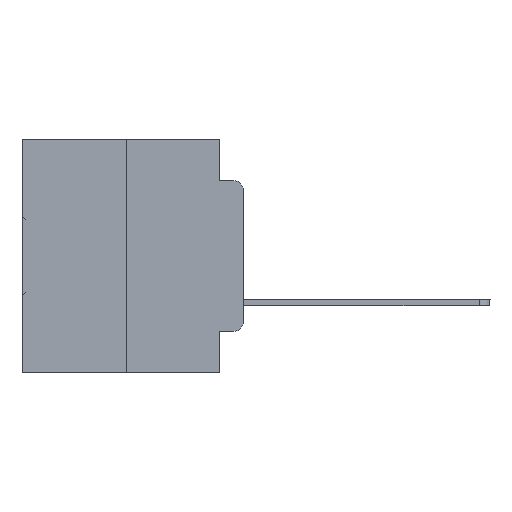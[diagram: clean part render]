
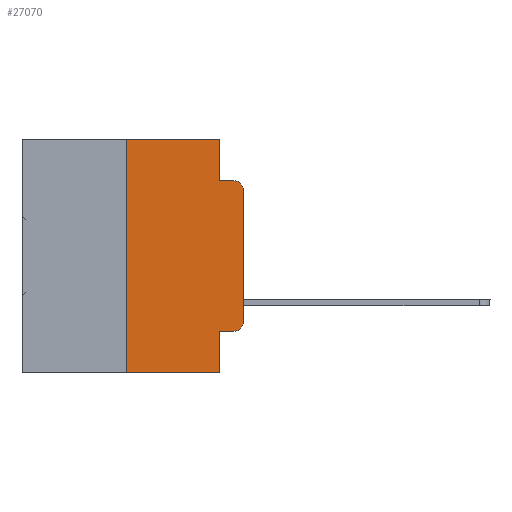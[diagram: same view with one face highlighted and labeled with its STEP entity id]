
A CAD part, left-side view. The second image highlights one B-rep face of the part: STEP entity #27070.
In plain terms, the highlighted planar face has unit normal (-1, 0, 0).
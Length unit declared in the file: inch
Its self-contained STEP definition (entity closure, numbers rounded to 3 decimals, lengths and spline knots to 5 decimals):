
#1309 = VERTEX_POINT ( 'NONE', #2288 ) ;
#1622 = DIRECTION ( 'NONE',  ( 0., 0., -1. ) ) ;
#1757 = EDGE_CURVE ( 'NONE', #30433, #1309, #8278, .T. ) ;
#2015 = VECTOR ( 'NONE', #1622, 39.37008 ) ;
#2288 = CARTESIAN_POINT ( 'NONE',  ( 0., 0.02, -0.0885 ) ) ;
#2417 = DIRECTION ( 'NONE',  ( 0., 0., 1. ) ) ;
#2540 = CARTESIAN_POINT ( 'NONE',  ( 0., 0.051, -0.4115 ) ) ;
#3320 = CARTESIAN_POINT ( 'NONE',  ( 0., 0.051, -0.0885 ) ) ;
#4092 = VECTOR ( 'NONE', #8995, 39.37008 ) ;
#4436 = CARTESIAN_POINT ( 'NONE',  ( 0., 0.25, 0. ) ) ;
#4823 = PLANE ( 'NONE',  #31212 ) ;
#6303 = ORIENTED_EDGE ( 'NONE', *, *, #8604, .T. ) ;
#6358 = CARTESIAN_POINT ( 'NONE',  ( 0., 0.02, -0.4115 ) ) ;
#7076 = CARTESIAN_POINT ( 'NONE',  ( 0., 0.051, -0.4115 ) ) ;
#7178 = LINE ( 'NONE', #12905, #24409 ) ;
#7400 = ORIENTED_EDGE ( 'NONE', *, *, #1757, .F. ) ;
#7734 = DIRECTION ( 'NONE',  ( 1., 0., 0. ) ) ;
#8064 = CARTESIAN_POINT ( 'NONE',  ( 0., 0.02, -0.3915 ) ) ;
#8278 = LINE ( 'NONE', #13047, #28483 ) ;
#8604 = EDGE_CURVE ( 'NONE', #26953, #14806, #32499, .T. ) ;
#8995 = DIRECTION ( 'NONE',  ( 0., -1., 0. ) ) ;
#9175 = VECTOR ( 'NONE', #30974, 39.37008 ) ;
#10134 = DIRECTION ( 'NONE',  ( 0., 0., -1. ) ) ;
#10216 = LINE ( 'NONE', #17256, #14032 ) ;
#10469 = DIRECTION ( 'NONE',  ( 0., 0., -1. ) ) ;
#11031 = ORIENTED_EDGE ( 'NONE', *, *, #35385, .T. ) ;
#11082 = DIRECTION ( 'NONE',  ( -1., 0., 0. ) ) ;
#12021 = ORIENTED_EDGE ( 'NONE', *, *, #30233, .F. ) ;
#12734 = EDGE_CURVE ( 'NONE', #35328, #30433, #23080, .T. ) ;
#12905 = CARTESIAN_POINT ( 'NONE',  ( 0., 0.25, 0. ) ) ;
#13047 = CARTESIAN_POINT ( 'NONE',  ( 0., 0.051, -0.0885 ) ) ;
#13958 = DIRECTION ( 'NONE',  ( 0., 0., -1. ) ) ;
#14032 = VECTOR ( 'NONE', #14249, 39.37008 ) ;
#14189 = VERTEX_POINT ( 'NONE', #4436 ) ;
#14249 = DIRECTION ( 'NONE',  ( 0., 0., -1. ) ) ;
#14806 = VERTEX_POINT ( 'NONE', #26949 ) ;
#15816 = EDGE_CURVE ( 'NONE', #33983, #16895, #25322, .T. ) ;
#15848 = ORIENTED_EDGE ( 'NONE', *, *, #16997, .F. ) ;
#16237 = LINE ( 'NONE', #2540, #27840 ) ;
#16338 = CARTESIAN_POINT ( 'NONE',  ( 0., 0.051, 0. ) ) ;
#16895 = VERTEX_POINT ( 'NONE', #29332 ) ;
#16997 = EDGE_CURVE ( 'NONE', #17046, #16895, #10216, .T. ) ;
#17046 = VERTEX_POINT ( 'NONE', #7076 ) ;
#17256 = CARTESIAN_POINT ( 'NONE',  ( 0., 0.051, 0. ) ) ;
#18840 = FACE_OUTER_BOUND ( 'NONE', #24145, .T. ) ;
#19273 = ORIENTED_EDGE ( 'NONE', *, *, #30307, .T. ) ;
#19648 = ORIENTED_EDGE ( 'NONE', *, *, #30508, .F. ) ;
#20889 = CARTESIAN_POINT ( 'NONE',  ( 0., 0.473, 0. ) ) ;
#21616 = CARTESIAN_POINT ( 'NONE',  ( 0., 0., -0.1085 ) ) ;
#21869 = DIRECTION ( 'NONE',  ( 0., -1., 0. ) ) ;
#22192 = ORIENTED_EDGE ( 'NONE', *, *, #15816, .T. ) ;
#22555 = LINE ( 'NONE', #28274, #4092 ) ;
#22891 = AXIS2_PLACEMENT_3D ( 'NONE', #24795, #11082, #13958 ) ;
#23013 = VERTEX_POINT ( 'NONE', #21616 ) ;
#23080 = LINE ( 'NONE', #31875, #2015 ) ;
#23506 = CARTESIAN_POINT ( 'NONE',  ( 0., 0.473, -0.5 ) ) ;
#24122 = CARTESIAN_POINT ( 'NONE',  ( 0., 0.25, -0.5 ) ) ;
#24145 = EDGE_LOOP ( 'NONE', ( #11031, #28302, #7400, #32050, #19648, #12021, #22192, #15848, #19273, #6303 ) ) ;
#24409 = VECTOR ( 'NONE', #2417, 39.37008 ) ;
#24795 = CARTESIAN_POINT ( 'NONE',  ( 0., 0.02, -0.1085 ) ) ;
#25196 = CARTESIAN_POINT ( 'NONE',  ( 0., 0., 0. ) ) ;
#25322 = LINE ( 'NONE', #23506, #29696 ) ;
#26949 = CARTESIAN_POINT ( 'NONE',  ( 0., 0., -0.3915 ) ) ;
#26953 = VERTEX_POINT ( 'NONE', #6358 ) ;
#27064 = DIRECTION ( 'NONE',  ( -1., 0., 0. ) ) ;
#27070 = ADVANCED_FACE ( 'NONE', ( #18840 ), #4823, .F. ) ;
#27840 = VECTOR ( 'NONE', #21869, 39.37008 ) ;
#27979 = CIRCLE ( 'NONE', #22891, 0.02 ) ;
#28192 = DIRECTION ( 'NONE',  ( 0., -1., 0. ) ) ;
#28208 = DIRECTION ( 'NONE',  ( 0., -1., 0. ) ) ;
#28274 = CARTESIAN_POINT ( 'NONE',  ( 0., 0.473, 0. ) ) ;
#28302 = ORIENTED_EDGE ( 'NONE', *, *, #28524, .T. ) ;
#28483 = VECTOR ( 'NONE', #28192, 39.37008 ) ;
#28524 = EDGE_CURVE ( 'NONE', #23013, #1309, #27979, .T. ) ;
#28889 = AXIS2_PLACEMENT_3D ( 'NONE', #8064, #27064, #10469 ) ;
#29332 = CARTESIAN_POINT ( 'NONE',  ( 0., 0.051, -0.5 ) ) ;
#29696 = VECTOR ( 'NONE', #28208, 39.37008 ) ;
#30233 = EDGE_CURVE ( 'NONE', #33983, #14189, #7178, .T. ) ;
#30307 = EDGE_CURVE ( 'NONE', #17046, #26953, #16237, .T. ) ;
#30433 = VERTEX_POINT ( 'NONE', #3320 ) ;
#30508 = EDGE_CURVE ( 'NONE', #14189, #35328, #22555, .T. ) ;
#30974 = DIRECTION ( 'NONE',  ( 0., 0., 1. ) ) ;
#31140 = LINE ( 'NONE', #25196, #9175 ) ;
#31212 = AXIS2_PLACEMENT_3D ( 'NONE', #20889, #7734, #10134 ) ;
#31875 = CARTESIAN_POINT ( 'NONE',  ( 0., 0.051, 0. ) ) ;
#32050 = ORIENTED_EDGE ( 'NONE', *, *, #12734, .F. ) ;
#32499 = CIRCLE ( 'NONE', #28889, 0.02 ) ;
#33983 = VERTEX_POINT ( 'NONE', #24122 ) ;
#35328 = VERTEX_POINT ( 'NONE', #16338 ) ;
#35385 = EDGE_CURVE ( 'NONE', #14806, #23013, #31140, .T. ) ;
